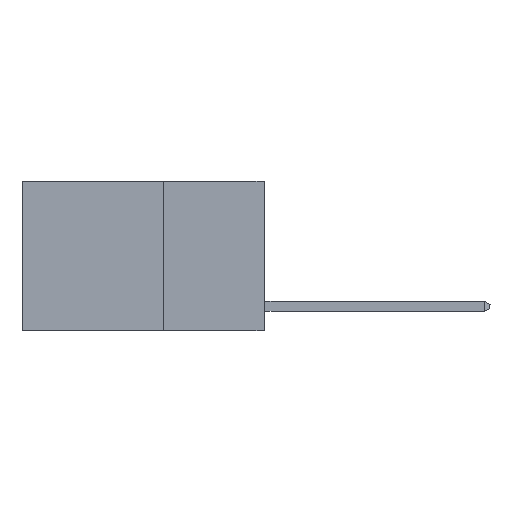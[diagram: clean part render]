
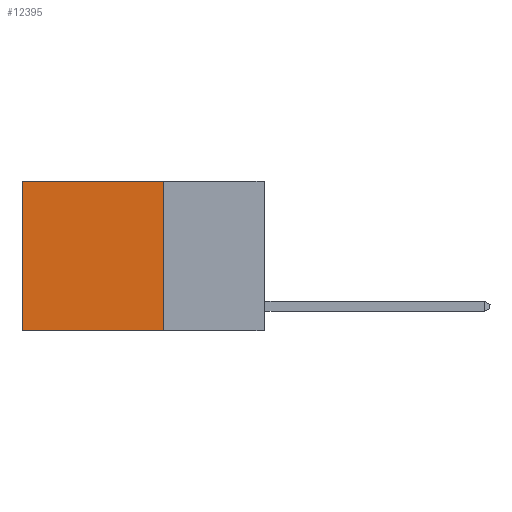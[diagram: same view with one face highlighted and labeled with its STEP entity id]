
A CAD part, left-side view. The second image highlights one B-rep face of the part: STEP entity #12395.
In plain terms, the highlighted planar face has unit normal (-1, 0, 0).
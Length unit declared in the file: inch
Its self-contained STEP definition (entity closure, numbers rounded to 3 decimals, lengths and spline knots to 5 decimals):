
#605 = VERTEX_POINT ( 'NONE', #2650 ) ;
#1692 = DIRECTION ( 'NONE',  ( 0., 0., -1. ) ) ;
#1925 = VECTOR ( 'NONE', #8317, 39.37008 ) ;
#1944 = EDGE_CURVE ( 'NONE', #14733, #605, #17681, .T. ) ;
#2090 = VERTEX_POINT ( 'NONE', #15681 ) ;
#2650 = CARTESIAN_POINT ( 'NONE',  ( 0.2625, 0.6, 0. ) ) ;
#3221 = FACE_OUTER_BOUND ( 'NONE', #7233, .T. ) ;
#3845 = LINE ( 'NONE', #12122, #17596 ) ;
#5071 = DIRECTION ( 'NONE',  ( 0., 0., -1. ) ) ;
#5095 = CARTESIAN_POINT ( 'NONE',  ( 0.2625, 0.25, -0.37 ) ) ;
#5130 = ORIENTED_EDGE ( 'NONE', *, *, #1944, .T. ) ;
#5163 = LINE ( 'NONE', #10815, #10800 ) ;
#5929 = CARTESIAN_POINT ( 'NONE',  ( 0.2625, 0.25, 0. ) ) ;
#6147 = LINE ( 'NONE', #10341, #8005 ) ;
#6652 = ORIENTED_EDGE ( 'NONE', *, *, #11008, .F. ) ;
#7203 = CARTESIAN_POINT ( 'NONE',  ( 0.2625, 0.25, 0. ) ) ;
#7233 = EDGE_LOOP ( 'NONE', ( #11565, #10759, #6652, #5130 ) ) ;
#7447 = EDGE_CURVE ( 'NONE', #13546, #2090, #6147, .T. ) ;
#8005 = VECTOR ( 'NONE', #14472, 39.37008 ) ;
#8317 = DIRECTION ( 'NONE',  ( 0., 1., 0. ) ) ;
#10341 = CARTESIAN_POINT ( 'NONE',  ( 0.2625, 0.25, -0.37 ) ) ;
#10759 = ORIENTED_EDGE ( 'NONE', *, *, #7447, .F. ) ;
#10800 = VECTOR ( 'NONE', #5071, 39.37008 ) ;
#10815 = CARTESIAN_POINT ( 'NONE',  ( 0.2625, 0.6, 0. ) ) ;
#10858 = DIRECTION ( 'NONE',  ( 0., 0., -1. ) ) ;
#11008 = EDGE_CURVE ( 'NONE', #14733, #13546, #3845, .T. ) ;
#11565 = ORIENTED_EDGE ( 'NONE', *, *, #17177, .T. ) ;
#12122 = CARTESIAN_POINT ( 'NONE',  ( 0.2625, 0.25, 0. ) ) ;
#12395 = ADVANCED_FACE ( 'NONE', ( #3221 ), #16639, .F. ) ;
#13522 = AXIS2_PLACEMENT_3D ( 'NONE', #5929, #13910, #1692 ) ;
#13546 = VERTEX_POINT ( 'NONE', #5095 ) ;
#13683 = CARTESIAN_POINT ( 'NONE',  ( 0.2625, 0.25, 0. ) ) ;
#13910 = DIRECTION ( 'NONE',  ( 1., 0., 0. ) ) ;
#14472 = DIRECTION ( 'NONE',  ( 0., 1., 0. ) ) ;
#14733 = VERTEX_POINT ( 'NONE', #7203 ) ;
#15681 = CARTESIAN_POINT ( 'NONE',  ( 0.2625, 0.6, -0.37 ) ) ;
#16639 = PLANE ( 'NONE',  #13522 ) ;
#17177 = EDGE_CURVE ( 'NONE', #605, #2090, #5163, .T. ) ;
#17596 = VECTOR ( 'NONE', #10858, 39.37008 ) ;
#17681 = LINE ( 'NONE', #13683, #1925 ) ;
